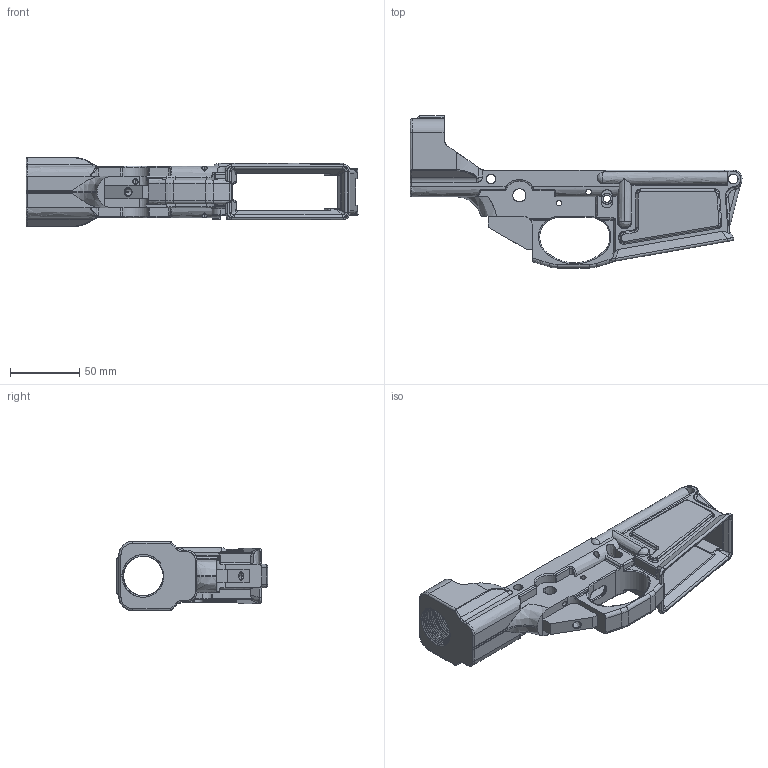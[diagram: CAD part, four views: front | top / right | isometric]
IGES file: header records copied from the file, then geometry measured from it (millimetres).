
Start section: SolidWorks IGES file using analytic representation for surfaces
Global section: file name: Nephilim_AR-10_V2.IGS; native system: SolidWorks 2015; preprocessor: SolidWorks 2015; author: WarFairy; date: 150516.234003; units: millimetre
Bounding box: 239.65 x 109.71 x 50 mm (x, y, z)
Surface area: 71001.3 mm2 (no closed solid volume)
Topology: 0 solids, 0 shells, 640 faces, 8208 edges, 8196 vertices
Faces by surface type: bspline 326, revolution 314
